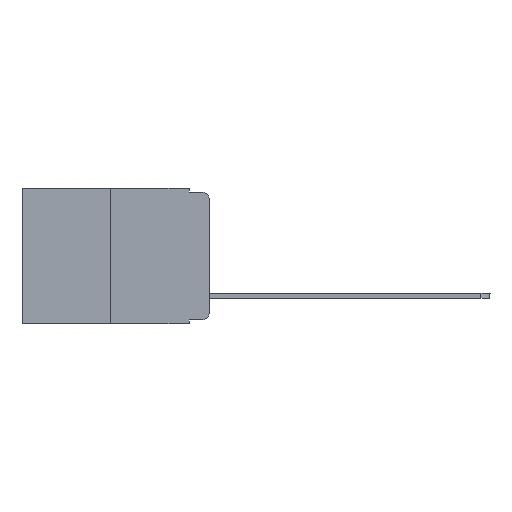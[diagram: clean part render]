
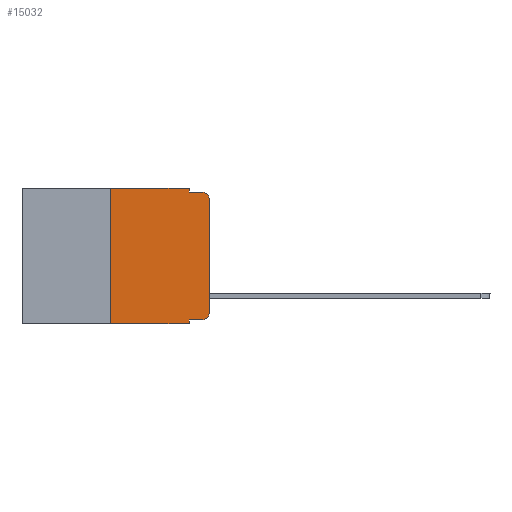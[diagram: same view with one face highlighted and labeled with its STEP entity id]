
A CAD part, left-side view. The second image highlights one B-rep face of the part: STEP entity #15032.
In plain terms, the highlighted planar face has unit normal (-1, 0, 0).
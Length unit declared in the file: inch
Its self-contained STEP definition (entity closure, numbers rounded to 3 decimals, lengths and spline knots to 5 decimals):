
#111 = ORIENTED_EDGE ( 'NONE', *, *, #19550, .T. ) ;
#604 = ORIENTED_EDGE ( 'NONE', *, *, #19182, .T. ) ;
#737 = EDGE_CURVE ( 'NONE', #759, #15093, #13238, .T. ) ;
#759 = VERTEX_POINT ( 'NONE', #2328 ) ;
#779 = CARTESIAN_POINT ( 'NONE',  ( 0., 0.02, -0.03 ) ) ;
#1097 = CARTESIAN_POINT ( 'NONE',  ( 0., 0., -0.313 ) ) ;
#1101 = CARTESIAN_POINT ( 'NONE',  ( 0., 0., 0. ) ) ;
#1284 = CARTESIAN_POINT ( 'NONE',  ( 0., 0.051, -0.01 ) ) ;
#1294 = CARTESIAN_POINT ( 'NONE',  ( 0., 0., -0.03 ) ) ;
#1905 = VECTOR ( 'NONE', #12850, 39.37008 ) ;
#1980 = CARTESIAN_POINT ( 'NONE',  ( 0., 0.051, 0. ) ) ;
#2328 = CARTESIAN_POINT ( 'NONE',  ( 0., 0.25, -0.343 ) ) ;
#2720 = VECTOR ( 'NONE', #7862, 39.37008 ) ;
#3008 = EDGE_CURVE ( 'NONE', #12077, #19323, #5316, .T. ) ;
#3776 = ORIENTED_EDGE ( 'NONE', *, *, #10554, .F. ) ;
#3797 = LINE ( 'NONE', #4718, #22263 ) ;
#3900 = EDGE_CURVE ( 'NONE', #11351, #10264, #15905, .T. ) ;
#3978 = VECTOR ( 'NONE', #15942, 39.37008 ) ;
#4718 = CARTESIAN_POINT ( 'NONE',  ( 0., 0.051, 0. ) ) ;
#4852 = ORIENTED_EDGE ( 'NONE', *, *, #18920, .T. ) ;
#5316 = LINE ( 'NONE', #18031, #10490 ) ;
#5341 = PLANE ( 'NONE',  #22025 ) ;
#5713 = CARTESIAN_POINT ( 'NONE',  ( 0., 0.02, -0.01 ) ) ;
#5727 = CARTESIAN_POINT ( 'NONE',  ( 0., 0.02, -0.333 ) ) ;
#6919 = DIRECTION ( 'NONE',  ( 0., 0., -1. ) ) ;
#7110 = DIRECTION ( 'NONE',  ( 0., -1., 0. ) ) ;
#7261 = ORIENTED_EDGE ( 'NONE', *, *, #737, .F. ) ;
#7315 = DIRECTION ( 'NONE',  ( 1., 0., 0. ) ) ;
#7336 = LINE ( 'NONE', #1980, #1905 ) ;
#7862 = DIRECTION ( 'NONE',  ( 0., 0., 1. ) ) ;
#8146 = CARTESIAN_POINT ( 'NONE',  ( 0., 0.02, -0.313 ) ) ;
#8982 = LINE ( 'NONE', #1101, #2720 ) ;
#9086 = DIRECTION ( 'NONE',  ( 0., -1., 0. ) ) ;
#9374 = DIRECTION ( 'NONE',  ( 0., 0., -1. ) ) ;
#9550 = DIRECTION ( 'NONE',  ( 0., -1., 0. ) ) ;
#10264 = VERTEX_POINT ( 'NONE', #5713 ) ;
#10437 = VERTEX_POINT ( 'NONE', #1294 ) ;
#10490 = VECTOR ( 'NONE', #9086, 39.37008 ) ;
#10554 = EDGE_CURVE ( 'NONE', #12077, #16894, #3797, .T. ) ;
#10866 = ORIENTED_EDGE ( 'NONE', *, *, #12853, .F. ) ;
#11035 = CARTESIAN_POINT ( 'NONE',  ( 0., 0.051, -0.343 ) ) ;
#11351 = VERTEX_POINT ( 'NONE', #14193 ) ;
#11796 = DIRECTION ( 'NONE',  ( 0., -1., 0. ) ) ;
#12077 = VERTEX_POINT ( 'NONE', #16044 ) ;
#12136 = VECTOR ( 'NONE', #9550, 39.37008 ) ;
#12262 = VECTOR ( 'NONE', #7110, 39.37008 ) ;
#12501 = DIRECTION ( 'NONE',  ( 0., 0., -1. ) ) ;
#12537 = CARTESIAN_POINT ( 'NONE',  ( 0., 0.25, 0. ) ) ;
#12850 = DIRECTION ( 'NONE',  ( 0., 0., -1. ) ) ;
#12853 = EDGE_CURVE ( 'NONE', #15093, #17900, #21319, .T. ) ;
#13107 = DIRECTION ( 'NONE',  ( 0., 0., -1. ) ) ;
#13238 = LINE ( 'NONE', #12537, #3978 ) ;
#14001 = VECTOR ( 'NONE', #11796, 39.37008 ) ;
#14025 = CARTESIAN_POINT ( 'NONE',  ( 0., 0.473, 0. ) ) ;
#14193 = CARTESIAN_POINT ( 'NONE',  ( 0., 0.051, -0.01 ) ) ;
#14598 = EDGE_CURVE ( 'NONE', #10437, #10264, #22201, .T. ) ;
#14961 = LINE ( 'NONE', #17506, #12262 ) ;
#15032 = ADVANCED_FACE ( 'NONE', ( #18983 ), #5341, .F. ) ;
#15093 = VERTEX_POINT ( 'NONE', #15839 ) ;
#15839 = CARTESIAN_POINT ( 'NONE',  ( 0., 0.25, 0. ) ) ;
#15905 = LINE ( 'NONE', #1284, #14001 ) ;
#15942 = DIRECTION ( 'NONE',  ( 0., 0., 1. ) ) ;
#16044 = CARTESIAN_POINT ( 'NONE',  ( 0., 0.051, -0.333 ) ) ;
#16442 = DIRECTION ( 'NONE',  ( -1., 0., 0. ) ) ;
#16481 = EDGE_LOOP ( 'NONE', ( #4852, #17605, #18166, #18949, #10866, #7261, #604, #3776, #19648, #111 ) ) ;
#16894 = VERTEX_POINT ( 'NONE', #11035 ) ;
#17179 = VERTEX_POINT ( 'NONE', #1097 ) ;
#17506 = CARTESIAN_POINT ( 'NONE',  ( 0., 0.473, -0.343 ) ) ;
#17605 = ORIENTED_EDGE ( 'NONE', *, *, #14598, .T. ) ;
#17900 = VERTEX_POINT ( 'NONE', #20966 ) ;
#18031 = CARTESIAN_POINT ( 'NONE',  ( 0., 0.051, -0.333 ) ) ;
#18056 = AXIS2_PLACEMENT_3D ( 'NONE', #8146, #20052, #13107 ) ;
#18166 = ORIENTED_EDGE ( 'NONE', *, *, #3900, .F. ) ;
#18352 = CARTESIAN_POINT ( 'NONE',  ( 0., 0.473, 0. ) ) ;
#18920 = EDGE_CURVE ( 'NONE', #17179, #10437, #8982, .T. ) ;
#18949 = ORIENTED_EDGE ( 'NONE', *, *, #21527, .F. ) ;
#18983 = FACE_OUTER_BOUND ( 'NONE', #16481, .T. ) ;
#19182 = EDGE_CURVE ( 'NONE', #759, #16894, #14961, .T. ) ;
#19323 = VERTEX_POINT ( 'NONE', #5727 ) ;
#19550 = EDGE_CURVE ( 'NONE', #19323, #17179, #20625, .T. ) ;
#19648 = ORIENTED_EDGE ( 'NONE', *, *, #3008, .T. ) ;
#20052 = DIRECTION ( 'NONE',  ( -1., 0., 0. ) ) ;
#20441 = AXIS2_PLACEMENT_3D ( 'NONE', #779, #16442, #9374 ) ;
#20625 = CIRCLE ( 'NONE', #18056, 0.02 ) ;
#20966 = CARTESIAN_POINT ( 'NONE',  ( 0., 0.051, 0. ) ) ;
#21319 = LINE ( 'NONE', #18352, #12136 ) ;
#21527 = EDGE_CURVE ( 'NONE', #17900, #11351, #7336, .T. ) ;
#22025 = AXIS2_PLACEMENT_3D ( 'NONE', #14025, #7315, #12501 ) ;
#22201 = CIRCLE ( 'NONE', #20441, 0.02 ) ;
#22263 = VECTOR ( 'NONE', #6919, 39.37008 ) ;
